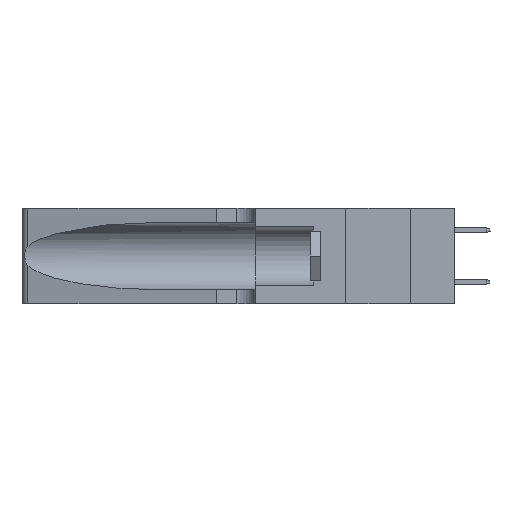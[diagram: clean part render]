
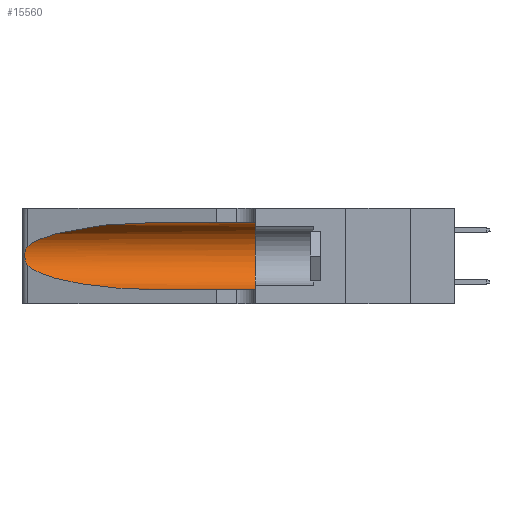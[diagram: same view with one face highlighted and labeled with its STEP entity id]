
A CAD part, left-side view. The second image highlights one B-rep face of the part: STEP entity #15560.
In plain terms, the highlighted cylindrical face has radius 3.308 mm (diameter 6.617 mm), a partial arc.
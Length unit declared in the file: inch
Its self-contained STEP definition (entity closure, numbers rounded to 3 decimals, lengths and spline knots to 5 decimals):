
#260 = VERTEX_POINT ( 'NONE', #18387 ) ;
#1271 = ORIENTED_EDGE ( 'NONE', *, *, #3692, .T. ) ;
#1283 = CARTESIAN_POINT ( 'NONE',  ( 0.26075, 1.23896, 0.178 ) ) ;
#1671 = CARTESIAN_POINT ( 'NONE',  ( 0.25487, 1.22718, 0.22369 ) ) ;
#1891 = ORIENTED_EDGE ( 'NONE', *, *, #19704, .T. ) ;
#2464 = CARTESIAN_POINT ( 'NONE',  ( 0.1305, 0.72297, 0.31525 ) ) ;
#3167 = CARTESIAN_POINT ( 'NONE',  ( 0.25487, 1.22718, 0.22369 ) ) ;
#3692 = EDGE_CURVE ( 'NONE', #19697, #260, #26119, .T. ) ;
#3814 = CARTESIAN_POINT ( 'NONE',  ( 0.1305, 1.61858, 0.05475 ) ) ;
#4014 = EDGE_CURVE ( 'NONE', #34943, #19697, #30151, .T. ) ;
#4393 = CARTESIAN_POINT ( 'NONE',  ( 0.1305, 1.61858, 0.185 ) ) ;
#4544 = CARTESIAN_POINT ( 'NONE',  ( 0.26018, 1.23835, 0.19895 ) ) ;
#6326 = LINE ( 'NONE', #3814, #37770 ) ;
#6726 = ORIENTED_EDGE ( 'NONE', *, *, #26128, .F. ) ;
#7075 = CARTESIAN_POINT ( 'NONE',  ( 0.1305, 0.35, 0.05475 ) ) ;
#7115 = AXIS2_PLACEMENT_3D ( 'NONE', #4393, #25002, #10382 ) ;
#7164 = CARTESIAN_POINT ( 'NONE',  ( 0.18966, 0.96281, 0.05475 ) ) ;
#7263 = CARTESIAN_POINT ( 'NONE',  ( 0.25787, 1.23484, 0.2124 ) ) ;
#7330 = EDGE_CURVE ( 'NONE', #35758, #34943, #19754, .T. ) ;
#7446 = CARTESIAN_POINT ( 'NONE',  ( 0.25487, 1.22718, 0.14631 ) ) ;
#9320 = ORIENTED_EDGE ( 'NONE', *, *, #11751, .F. ) ;
#9850 = CARTESIAN_POINT ( 'NONE',  ( 0.25487, 1.22718, 0.22369 ) ) ;
#10382 = DIRECTION ( 'NONE',  ( 0., 0., -1. ) ) ;
#11751 = EDGE_CURVE ( 'NONE', #35758, #19480, #31315, .T. ) ;
#12182 = CARTESIAN_POINT ( 'NONE',  ( 0.1305, 0.72297, 0.31525 ) ) ;
#13114 = CARTESIAN_POINT ( 'NONE',  ( 0.1305, 0.72297, 0.05475 ) ) ;
#13134 = DIRECTION ( 'NONE',  ( 0., 1., 0. ) ) ;
#13251 = CYLINDRICAL_SURFACE ( 'NONE', #7115, 0.13025 ) ;
#13333 = CARTESIAN_POINT ( 'NONE',  ( 0.1305, 0.35, 0.31525 ) ) ;
#13517 = CARTESIAN_POINT ( 'NONE',  ( 0.1305, 0.35, 0.185 ) ) ;
#13595 = CARTESIAN_POINT ( 'NONE',  ( 0.25854, 1.2359, 0.20912 ) ) ;
#14284 = DIRECTION ( 'NONE',  ( 0., -1., 0. ) ) ;
#14288 = VERTEX_POINT ( 'NONE', #7075 ) ;
#15069 = CARTESIAN_POINT ( 'NONE',  ( 0.2373, 1.15595, 0.28018 ) ) ;
#15560 = ADVANCED_FACE ( 'NONE', ( #30750 ), #13251, .F. ) ;
#15724 = CARTESIAN_POINT ( 'NONE',  ( 0.25555, 1.22993, 0.14849 ) ) ;
#15820 = CARTESIAN_POINT ( 'NONE',  ( 0.25487, 1.22718, 0.14631 ) ) ;
#16476 = CARTESIAN_POINT ( 'NONE',  ( 0.25555, 1.22994, 0.2215 ) ) ;
#18387 = CARTESIAN_POINT ( 'NONE',  ( 0.1305, 0.72297, 0.05475 ) ) ;
#19480 = VERTEX_POINT ( 'NONE', #13333 ) ;
#19697 = VERTEX_POINT ( 'NONE', #27111 ) ;
#19704 = EDGE_CURVE ( 'NONE', #260, #14288, #6326, .T. ) ;
#19754 =( BOUNDED_CURVE ( )  B_SPLINE_CURVE ( 3, ( #12182, #30425, #15069, #9850 ),
 .UNSPECIFIED., .F., .T. ) 
 B_SPLINE_CURVE_WITH_KNOTS ( ( 4, 4 ),
 ( 1.5708, 2.84003 ),
 .UNSPECIFIED. ) 
 CURVE ( )  GEOMETRIC_REPRESENTATION_ITEM ( )  RATIONAL_B_SPLINE_CURVE ( ( 1., 0.87, 0.87, 1. ) ) 
 REPRESENTATION_ITEM ( '' )  );
#21790 = CARTESIAN_POINT ( 'NONE',  ( 0.2373, 1.15595, 0.08982 ) ) ;
#21888 = CARTESIAN_POINT ( 'NONE',  ( 0.25856, 1.23593, 0.16098 ) ) ;
#22072 = CARTESIAN_POINT ( 'NONE',  ( 0.25789, 1.23486, 0.15765 ) ) ;
#22461 = DIRECTION ( 'NONE',  ( 0., -1., 0. ) ) ;
#24581 = CARTESIAN_POINT ( 'NONE',  ( 0.26017, 1.23833, 0.17102 ) ) ;
#25002 = DIRECTION ( 'NONE',  ( 0., -1., 0. ) ) ;
#25153 = CARTESIAN_POINT ( 'NONE',  ( 0.25639, 1.23184, 0.21858 ) ) ;
#25291 = ORIENTED_EDGE ( 'NONE', *, *, #4014, .T. ) ;
#25342 = CARTESIAN_POINT ( 'NONE',  ( 0.25639, 1.23186, 0.15144 ) ) ;
#26119 =( BOUNDED_CURVE ( )  B_SPLINE_CURVE ( 3, ( #15820, #21790, #7164, #13114 ),
 .UNSPECIFIED., .F., .T. ) 
 B_SPLINE_CURVE_WITH_KNOTS ( ( 4, 4 ),
 ( 3.44316, 4.71239 ),
 .UNSPECIFIED. ) 
 CURVE ( )  GEOMETRIC_REPRESENTATION_ITEM ( )  RATIONAL_B_SPLINE_CURVE ( ( 1., 0.87, 0.87, 1. ) ) 
 REPRESENTATION_ITEM ( '' )  );
#26128 = EDGE_CURVE ( 'NONE', #19480, #14288, #35443, .T. ) ;
#27111 = CARTESIAN_POINT ( 'NONE',  ( 0.25487, 1.22718, 0.14631 ) ) ;
#27469 = CARTESIAN_POINT ( 'NONE',  ( 0.26075, 1.23896, 0.19203 ) ) ;
#28086 = VECTOR ( 'NONE', #22461, 39.37008 ) ;
#29923 = AXIS2_PLACEMENT_3D ( 'NONE', #13517, #13134, #31015 ) ;
#30151 = B_SPLINE_CURVE_WITH_KNOTS ( 'NONE', 3,
 ( #1671, #16476, #25153, #7263, #13595, #4544, #27469, #1283, #24581, #21888, #22072, #25342, #15724, #7446 ),
 .UNSPECIFIED., .F., .F.,
 ( 4, 2, 2, 2, 2, 2, 4 ),
 ( 0., 0.00027, 0.00053, 0.00107, 0.0016, 0.00187, 0.00214 ),
 .UNSPECIFIED. ) ;
#30419 = EDGE_LOOP ( 'NONE', ( #35737, #25291, #1271, #1891, #6726, #9320 ) ) ;
#30425 = CARTESIAN_POINT ( 'NONE',  ( 0.18966, 0.96281, 0.31525 ) ) ;
#30750 = FACE_OUTER_BOUND ( 'NONE', #30419, .T. ) ;
#31015 = DIRECTION ( 'NONE',  ( 0., 0., 1. ) ) ;
#31315 = LINE ( 'NONE', #31693, #28086 ) ;
#31693 = CARTESIAN_POINT ( 'NONE',  ( 0.1305, 1.61858, 0.31525 ) ) ;
#34943 = VERTEX_POINT ( 'NONE', #3167 ) ;
#35443 = CIRCLE ( 'NONE', #29923, 0.13025 ) ;
#35737 = ORIENTED_EDGE ( 'NONE', *, *, #7330, .T. ) ;
#35758 = VERTEX_POINT ( 'NONE', #2464 ) ;
#37770 = VECTOR ( 'NONE', #14284, 39.37008 ) ;
